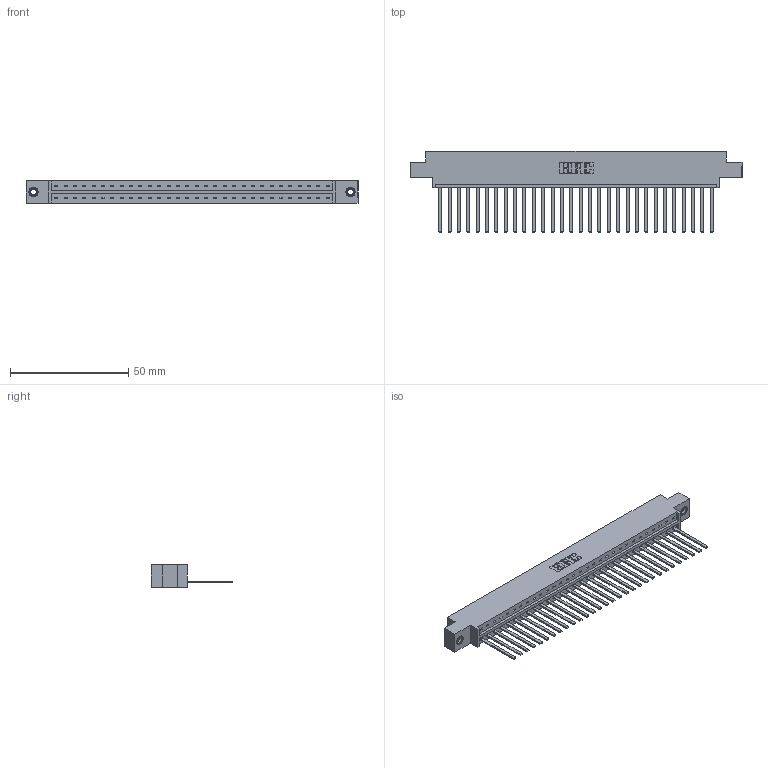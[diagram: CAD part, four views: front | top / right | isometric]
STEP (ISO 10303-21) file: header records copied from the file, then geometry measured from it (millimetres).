
FILE_DESCRIPTION (( 'STEP AP203' ), '1' );
FILE_NAME ('833-030-544-607.STEP', '2020-06-02T13:49:05', ( '' ), ( '' ), 'SwSTEP 2.0', 'SolidWorks 2020', '' );
FILE_SCHEMA (( 'CONFIG_CONTROL_DESIGN' ));
Length unit declared in the file: inch
Products named in the file (4): 833-030-544-607; 345-292-001_345-293-144; 345-250-001_345-250-005-103; 833 Part_Offset - .156 Dia - TI
Assembly tree (33 placements, depth 2):
  833-030-544-607
    833 Part_Offset - .156 Dia - TI
    345-292-001_345-293-144  x30
    345-250-001_345-250-005-103  x2
Bounding box: 140.41 x 34.3 x 9.4 mm (x, y, z)
Volume: 14132.3 mm3; surface area: 16577.6 mm2
Topology: 33 solids, 33 shells, 1738 faces, 5199 edges, 3418 vertices
Faces by surface type: plane 1246, cylinder 476, cone 12, torus 4
Entity records: 21026 total; most frequent: CARTESIAN_POINT 3611, ORIENTED_EDGE 3570, DIRECTION 3099, EDGE_CURVE 1785, LINE 1641, VECTOR 1641, VERTEX_POINT 1184, AXIS2_PLACEMENT_3D 729
